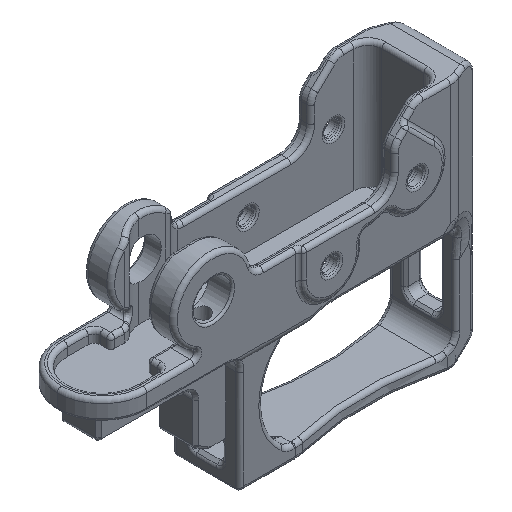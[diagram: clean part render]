
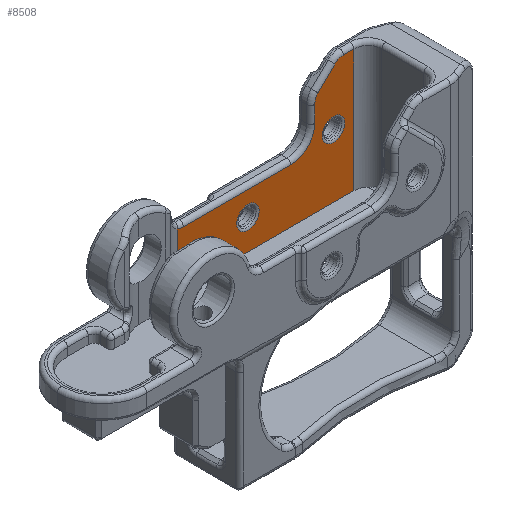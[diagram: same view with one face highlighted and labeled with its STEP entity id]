
A CAD part, isometric view. The second image highlights one B-rep face of the part: STEP entity #8508.
In plain terms, the highlighted planar face has unit normal (0, -1, 0).
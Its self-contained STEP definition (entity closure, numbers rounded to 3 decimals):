
#165=FACE_BOUND('',#2393,.T.);
#166=FACE_BOUND('',#2394,.T.);
#451=PLANE('',#9249);
#674=LINE('',#14311,#1162);
#690=LINE('',#14403,#1178);
#741=LINE('',#14614,#1229);
#742=LINE('',#14616,#1230);
#743=LINE('',#14620,#1231);
#744=LINE('',#14624,#1232);
#745=LINE('',#14628,#1233);
#1162=VECTOR('',#10738,10.);
#1178=VECTOR('',#10792,10.);
#1229=VECTOR('',#10971,10.);
#1230=VECTOR('',#10972,10.);
#1231=VECTOR('',#10975,10.);
#1232=VECTOR('',#10978,10.);
#1233=VECTOR('',#10981,10.);
#1832=FACE_OUTER_BOUND('',#2392,.T.);
#2392=EDGE_LOOP('',(#6412,#6413,#6414,#6415,#6416,#6417,#6418,#6419,#6420,
#6421,#6422));
#2393=EDGE_LOOP('',(#6423));
#2394=EDGE_LOOP('',(#6424));
#2963=CIRCLE('',#9247,2.811);
#2965=CIRCLE('',#9250,3.);
#2966=CIRCLE('',#9251,3.);
#2967=CIRCLE('',#9252,6.);
#2968=CIRCLE('',#9253,4.);
#2969=CIRCLE('',#9254,2.811);
#3648=VERTEX_POINT('',#14308);
#3649=VERTEX_POINT('',#14310);
#3682=VERTEX_POINT('',#14401);
#3730=VERTEX_POINT('',#14608);
#3731=VERTEX_POINT('',#14613);
#3732=VERTEX_POINT('',#14615);
#3733=VERTEX_POINT('',#14617);
#3734=VERTEX_POINT('',#14619);
#3735=VERTEX_POINT('',#14621);
#3736=VERTEX_POINT('',#14623);
#3737=VERTEX_POINT('',#14625);
#3738=VERTEX_POINT('',#14627);
#3739=VERTEX_POINT('',#14630);
#4562=EDGE_CURVE('',#3648,#3649,#674,.T.);
#4598=EDGE_CURVE('',#3682,#3648,#690,.T.);
#4681=EDGE_CURVE('',#3730,#3730,#2963,.T.);
#4683=EDGE_CURVE('',#3649,#3731,#741,.T.);
#4684=EDGE_CURVE('',#3732,#3682,#742,.T.);
#4685=EDGE_CURVE('',#3733,#3732,#2965,.T.);
#4686=EDGE_CURVE('',#3734,#3733,#743,.T.);
#4687=EDGE_CURVE('',#3735,#3734,#2966,.T.);
#4688=EDGE_CURVE('',#3736,#3735,#744,.T.);
#4689=EDGE_CURVE('',#3737,#3736,#2967,.T.);
#4690=EDGE_CURVE('',#3738,#3737,#745,.T.);
#4691=EDGE_CURVE('',#3731,#3738,#2968,.T.);
#4692=EDGE_CURVE('',#3739,#3739,#2969,.T.);
#6412=ORIENTED_EDGE('',*,*,#4683,.F.);
#6413=ORIENTED_EDGE('',*,*,#4562,.F.);
#6414=ORIENTED_EDGE('',*,*,#4598,.F.);
#6415=ORIENTED_EDGE('',*,*,#4684,.F.);
#6416=ORIENTED_EDGE('',*,*,#4685,.F.);
#6417=ORIENTED_EDGE('',*,*,#4686,.F.);
#6418=ORIENTED_EDGE('',*,*,#4687,.F.);
#6419=ORIENTED_EDGE('',*,*,#4688,.F.);
#6420=ORIENTED_EDGE('',*,*,#4689,.F.);
#6421=ORIENTED_EDGE('',*,*,#4690,.F.);
#6422=ORIENTED_EDGE('',*,*,#4691,.F.);
#6423=ORIENTED_EDGE('',*,*,#4692,.F.);
#6424=ORIENTED_EDGE('',*,*,#4681,.F.);
#8508=ADVANCED_FACE('',(#1832,#165,#166),#451,.T.);
#9247=AXIS2_PLACEMENT_3D('',#14610,#10965,#10966);
#9249=AXIS2_PLACEMENT_3D('',#14612,#10969,#10970);
#9250=AXIS2_PLACEMENT_3D('',#14618,#10973,#10974);
#9251=AXIS2_PLACEMENT_3D('',#14622,#10976,#10977);
#9252=AXIS2_PLACEMENT_3D('',#14626,#10979,#10980);
#9253=AXIS2_PLACEMENT_3D('',#14629,#10982,#10983);
#9254=AXIS2_PLACEMENT_3D('',#14631,#10984,#10985);
#10738=DIRECTION('',(-1.,0.,0.));
#10792=DIRECTION('',(0.,0.,-1.));
#10965=DIRECTION('center_axis',(0.,-1.,0.));
#10966=DIRECTION('ref_axis',(1.,0.,0.));
#10969=DIRECTION('center_axis',(0.,-1.,0.));
#10970=DIRECTION('ref_axis',(-1.,0.,0.));
#10971=DIRECTION('',(0.,0.,1.));
#10972=DIRECTION('',(1.,0.,0.));
#10973=DIRECTION('center_axis',(0.,1.,0.));
#10974=DIRECTION('ref_axis',(-0.383,0.,0.924));
#10975=DIRECTION('',(0.707,0.,0.707));
#10976=DIRECTION('center_axis',(0.,1.,0.));
#10977=DIRECTION('ref_axis',(-0.924,0.,0.383));
#10978=DIRECTION('',(0.,0.,1.));
#10979=DIRECTION('center_axis',(0.,-1.,0.));
#10980=DIRECTION('ref_axis',(0.707,0.,-0.707));
#10981=DIRECTION('',(1.,0.,0.));
#10982=DIRECTION('center_axis',(0.,-1.,0.));
#10983=DIRECTION('ref_axis',(-0.281,0.,-0.96));
#10984=DIRECTION('center_axis',(0.,-1.,0.));
#10985=DIRECTION('ref_axis',(1.,0.,0.));
#14308=CARTESIAN_POINT('',(-20.293,8.763,33.998));
#14310=CARTESIAN_POINT('',(-64.532,8.763,33.998));
#14311=CARTESIAN_POINT('',(-26.861,8.763,33.998));
#14401=CARTESIAN_POINT('',(-20.293,8.763,64.722));
#14403=CARTESIAN_POINT('',(-20.293,8.763,67.175));
#14608=CARTESIAN_POINT('',(-46.816,8.763,44.302));
#14610=CARTESIAN_POINT('Origin',(-46.816,8.763,41.491));
#14612=CARTESIAN_POINT('Origin',(-20.114,8.763,67.175));
#14613=CARTESIAN_POINT('',(-64.532,8.763,47.833));
#14614=CARTESIAN_POINT('',(-64.532,8.763,50.587));
#14615=CARTESIAN_POINT('',(-22.942,8.763,64.723));
#14616=CARTESIAN_POINT('',(24.981,8.763,64.722));
#14617=CARTESIAN_POINT('',(-25.064,8.763,63.844));
#14618=CARTESIAN_POINT('Origin',(-22.942,8.763,61.723));
#14619=CARTESIAN_POINT('',(-29.22,8.763,59.687));
#14620=CARTESIAN_POINT('',(-24.157,8.763,64.75));
#14621=CARTESIAN_POINT('',(-30.099,8.763,57.566));
#14622=CARTESIAN_POINT('Origin',(-27.099,8.763,57.566));
#14623=CARTESIAN_POINT('',(-30.099,8.763,53.491));
#14624=CARTESIAN_POINT('',(-30.099,8.763,62.341));
#14625=CARTESIAN_POINT('',(-36.099,8.763,47.491));
#14626=CARTESIAN_POINT('Origin',(-36.099,8.763,53.491));
#14627=CARTESIAN_POINT('',(-62.914,8.763,47.491));
#14628=CARTESIAN_POINT('',(-52.234,8.763,47.491));
#14629=CARTESIAN_POINT('Origin',(-62.914,8.763,51.491));
#14630=CARTESIAN_POINT('',(-25.403,8.763,52.658));
#14631=CARTESIAN_POINT('Origin',(-25.403,8.763,49.848));
